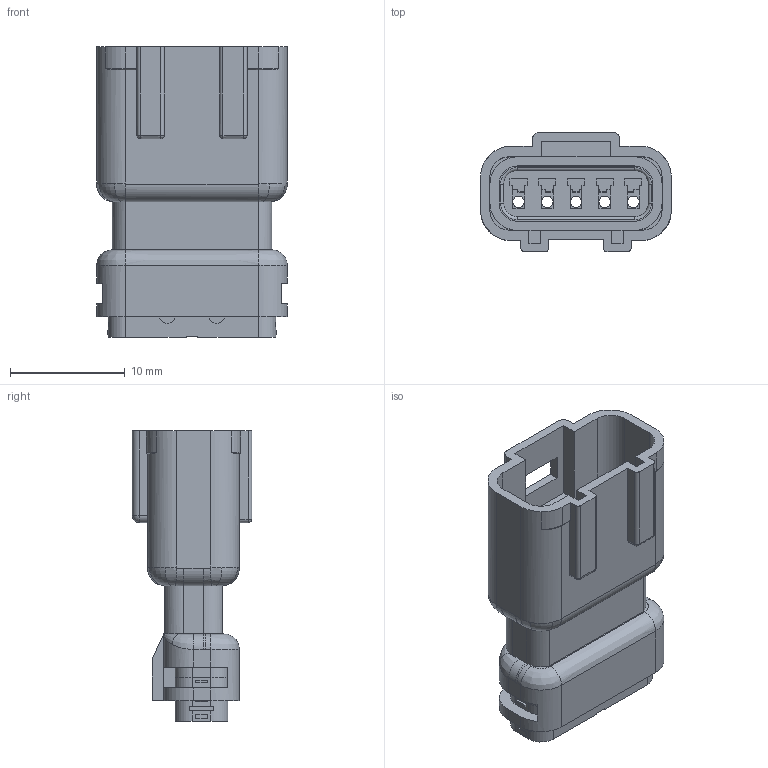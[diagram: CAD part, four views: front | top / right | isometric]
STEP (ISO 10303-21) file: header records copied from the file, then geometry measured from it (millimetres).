
FILE_DESCRIPTION (( 'STEP AP214' ), '1' );
FILE_NAME ('565-005-000-310.STEP', '2020-07-27T15:43:04', ( '' ), ( '' ), 'SwSTEP 2.0', 'SolidWorks 2020', '' );
FILE_SCHEMA (( 'AUTOMOTIVE_DESIGN' ));
Length unit declared in the file: millimetre
Products named in the file (5): 565-005-000-310_Rear Gasket; 565-005-000-310_Housing; 565-005-000-310_Rear Insulator; 565-005-000-310; 565-005-000-310_Front Gasket
Assembly tree (4 placements, depth 2):
  565-005-000-310
    565-005-000-310_Housing
    565-005-000-310_Rear Insulator
    565-005-000-310_Rear Gasket
    565-005-000-310_Front Gasket
Bounding box: 16.6 x 10.4 x 25.3 mm (x, y, z)
Volume: 1483.5 mm3; surface area: 3517.6 mm2
Topology: 4 solids, 4 shells, 610 faces, 1631 edges, 1052 vertices
Faces by surface type: plane 327, cylinder 175, bspline 58, torus 44, sphere 6
Entity records: 20755 total; most frequent: CARTESIAN_POINT 5497, ORIENTED_EDGE 3250, DIRECTION 3035, EDGE_CURVE 1625, VERTEX_POINT 1052, AXIS2_PLACEMENT_3D 1018, VECTOR 999, LINE 999
